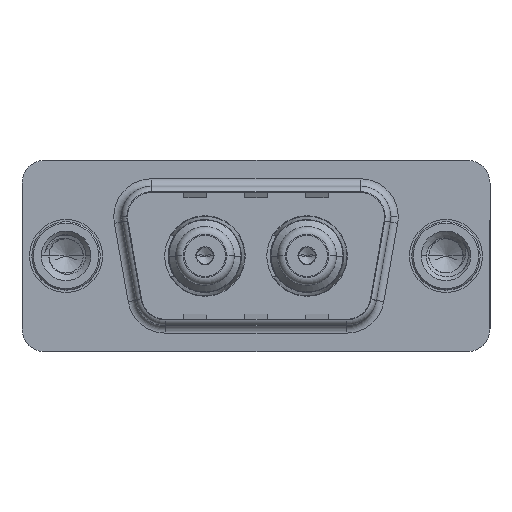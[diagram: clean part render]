
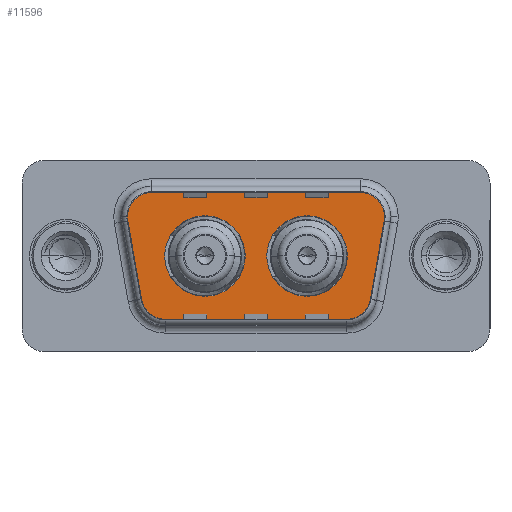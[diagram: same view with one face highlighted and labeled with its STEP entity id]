
A CAD part, top view. The second image highlights one B-rep face of the part: STEP entity #11596.
In plain terms, the highlighted planar face has unit normal (0, 0, 1).
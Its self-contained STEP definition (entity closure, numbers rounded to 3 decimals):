
#60 = DIRECTION ( 'NONE',  ( -1., 0., 0. ) ) ;
#128 = DIRECTION ( 'NONE',  ( 0., 0., 1. ) ) ;
#171 = AXIS2_PLACEMENT_3D ( 'NONE', #3546, #12994, #4929 ) ;
#443 = CARTESIAN_POINT ( 'NONE',  ( 6.459, -4.9, 0. ) ) ;
#576 = CARTESIAN_POINT ( 'NONE',  ( 5.436, 4.9, 0. ) ) ;
#838 = ORIENTED_EDGE ( 'NONE', *, *, #3028, .T. ) ;
#937 = DIRECTION ( 'NONE',  ( 0., 0., 1. ) ) ;
#1273 = DIRECTION ( 'NONE',  ( 0., 0., 1. ) ) ;
#1334 = ORIENTED_EDGE ( 'NONE', *, *, #12226, .F. ) ;
#1441 = VERTEX_POINT ( 'NONE', #5555 ) ;
#1493 = CARTESIAN_POINT ( 'NONE',  ( 20.511, -3.247, 0. ) ) ;
#1774 = ORIENTED_EDGE ( 'NONE', *, *, #13224, .F. ) ;
#1901 = PLANE ( 'NONE',  #8703 ) ;
#2397 = DIRECTION ( 'NONE',  ( 0., 0., 1. ) ) ;
#2769 = CIRCLE ( 'NONE', #3136, 2. ) ;
#2845 = VERTEX_POINT ( 'NONE', #7801 ) ;
#3028 = EDGE_CURVE ( 'NONE', #17390, #1441, #2769, .T. ) ;
#3136 = AXIS2_PLACEMENT_3D ( 'NONE', #5857, #11911, #10556 ) ;
#3280 = CARTESIAN_POINT ( 'NONE',  ( 13.21, 0., 0. ) ) ;
#3546 = CARTESIAN_POINT ( 'NONE',  ( 15.86, 0., 0. ) ) ;
#3594 = EDGE_LOOP ( 'NONE', ( #1774, #10455 ) ) ;
#3660 = ORIENTED_EDGE ( 'NONE', *, *, #9618, .T. ) ;
#4076 = DIRECTION ( 'NONE',  ( 0.174, 0.985, 0. ) ) ;
#4195 = EDGE_CURVE ( 'NONE', #12806, #14596, #5097, .T. ) ;
#4252 = VECTOR ( 'NONE', #12597, 1000. ) ;
#4644 = EDGE_CURVE ( 'NONE', #6173, #17390, #8700, .T. ) ;
#4682 = DIRECTION ( 'NONE',  ( 0., 0., 1. ) ) ;
#4697 = VERTEX_POINT ( 'NONE', #3280 ) ;
#4922 = VERTEX_POINT ( 'NONE', #5548 ) ;
#4929 = DIRECTION ( 'NONE',  ( 1., 0., 0. ) ) ;
#4947 = DIRECTION ( 'NONE',  ( 1., 0., 0. ) ) ;
#5097 = CIRCLE ( 'NONE', #16271, 2. ) ;
#5185 = ORIENTED_EDGE ( 'NONE', *, *, #14272, .T. ) ;
#5450 = EDGE_CURVE ( 'NONE', #14596, #13306, #6565, .T. ) ;
#5460 = CARTESIAN_POINT ( 'NONE',  ( 5.436, 4.9, 0. ) ) ;
#5471 = DIRECTION ( 'NONE',  ( 0.174, -0.985, 0. ) ) ;
#5548 = CARTESIAN_POINT ( 'NONE',  ( 6.459, -4.9, 0. ) ) ;
#5555 = CARTESIAN_POINT ( 'NONE',  ( 19.564, 4.9, 0. ) ) ;
#5847 = AXIS2_PLACEMENT_3D ( 'NONE', #14901, #6826, #16243 ) ;
#5849 = CIRCLE ( 'NONE', #14336, 2.65 ) ;
#5857 = CARTESIAN_POINT ( 'NONE',  ( 19.564, 2.9, 0. ) ) ;
#6173 = VERTEX_POINT ( 'NONE', #9937 ) ;
#6263 = CARTESIAN_POINT ( 'NONE',  ( 3.466, 2.553, 0. ) ) ;
#6487 = FACE_BOUND ( 'NONE', #13799, .T. ) ;
#6512 = ORIENTED_EDGE ( 'NONE', *, *, #14860, .F. ) ;
#6548 = LINE ( 'NONE', #576, #9695 ) ;
#6565 = LINE ( 'NONE', #12731, #9291 ) ;
#6826 = DIRECTION ( 'NONE',  ( 0., 0., 1. ) ) ;
#6878 = DIRECTION ( 'NONE',  ( 0., 0., 1. ) ) ;
#6931 = EDGE_CURVE ( 'NONE', #4922, #2845, #15038, .T. ) ;
#7434 = DIRECTION ( 'NONE',  ( -1., 0., 0. ) ) ;
#7801 = CARTESIAN_POINT ( 'NONE',  ( 18.541, -4.9, 0. ) ) ;
#7809 = VERTEX_POINT ( 'NONE', #1493 ) ;
#8114 = CIRCLE ( 'NONE', #5847, 2.65 ) ;
#8216 = VECTOR ( 'NONE', #4076, 1000. ) ;
#8343 = DIRECTION ( 'NONE',  ( 0., 0., 1. ) ) ;
#8403 = CARTESIAN_POINT ( 'NONE',  ( 15.86, 0., 0. ) ) ;
#8700 = CIRCLE ( 'NONE', #11063, 2. ) ;
#8703 = AXIS2_PLACEMENT_3D ( 'NONE', #11393, #4682, #14122 ) ;
#9019 = CARTESIAN_POINT ( 'NONE',  ( 5.436, 2.9, 0. ) ) ;
#9164 = CARTESIAN_POINT ( 'NONE',  ( 9.14, 0., 0. ) ) ;
#9187 = CARTESIAN_POINT ( 'NONE',  ( 4.489, -3.247, 0. ) ) ;
#9271 = CARTESIAN_POINT ( 'NONE',  ( 18.51, 0., 0. ) ) ;
#9291 = VECTOR ( 'NONE', #5471, 1000. ) ;
#9311 = EDGE_CURVE ( 'NONE', #1441, #12806, #6548, .T. ) ;
#9360 = CARTESIAN_POINT ( 'NONE',  ( 11.79, 0., 0. ) ) ;
#9487 = CARTESIAN_POINT ( 'NONE',  ( 18.541, -2.9, 0. ) ) ;
#9618 = EDGE_CURVE ( 'NONE', #2845, #7809, #17087, .T. ) ;
#9695 = VECTOR ( 'NONE', #7434, 1000. ) ;
#9727 = DIRECTION ( 'NONE',  ( 1., 0., 0. ) ) ;
#9844 = CARTESIAN_POINT ( 'NONE',  ( 21.564, 2.9, 0. ) ) ;
#9905 = ORIENTED_EDGE ( 'NONE', *, *, #6931, .T. ) ;
#9937 = CARTESIAN_POINT ( 'NONE',  ( 21.534, 2.553, 0. ) ) ;
#10294 = EDGE_CURVE ( 'NONE', #7809, #6173, #14941, .T. ) ;
#10455 = ORIENTED_EDGE ( 'NONE', *, *, #15374, .F. ) ;
#10480 = DIRECTION ( 'NONE',  ( 1., 0., 0. ) ) ;
#10542 = CIRCLE ( 'NONE', #14545, 2.65 ) ;
#10556 = DIRECTION ( 'NONE',  ( -1., 0., 0. ) ) ;
#10571 = CARTESIAN_POINT ( 'NONE',  ( 19.564, 2.9, 0. ) ) ;
#10816 = DIRECTION ( 'NONE',  ( 1., 0., 0. ) ) ;
#11060 = ORIENTED_EDGE ( 'NONE', *, *, #4195, .T. ) ;
#11063 = AXIS2_PLACEMENT_3D ( 'NONE', #10571, #6878, #16363 ) ;
#11270 = VERTEX_POINT ( 'NONE', #9360 ) ;
#11326 = CARTESIAN_POINT ( 'NONE',  ( 6.49, 0., 0. ) ) ;
#11393 = CARTESIAN_POINT ( 'NONE',  ( 18.541, -2.9, 0. ) ) ;
#11415 = ORIENTED_EDGE ( 'NONE', *, *, #4644, .T. ) ;
#11596 = ADVANCED_FACE ( 'NONE', ( #16792, #6487, #13192 ), #1901, .T. ) ;
#11909 = CIRCLE ( 'NONE', #171, 2.65 ) ;
#11911 = DIRECTION ( 'NONE',  ( 0., 0., 1. ) ) ;
#12162 = CARTESIAN_POINT ( 'NONE',  ( 21.534, 2.553, 0. ) ) ;
#12226 = EDGE_CURVE ( 'NONE', #15119, #11270, #5849, .T. ) ;
#12597 = DIRECTION ( 'NONE',  ( 1., 0., 0. ) ) ;
#12731 = CARTESIAN_POINT ( 'NONE',  ( 3.466, 2.553, 0. ) ) ;
#12806 = VERTEX_POINT ( 'NONE', #5460 ) ;
#12994 = DIRECTION ( 'NONE',  ( 0., 0., 1. ) ) ;
#13192 = FACE_OUTER_BOUND ( 'NONE', #16115, .T. ) ;
#13224 = EDGE_CURVE ( 'NONE', #14132, #4697, #11909, .T. ) ;
#13306 = VERTEX_POINT ( 'NONE', #9187 ) ;
#13429 = ORIENTED_EDGE ( 'NONE', *, *, #5450, .T. ) ;
#13799 = EDGE_LOOP ( 'NONE', ( #6512, #1334 ) ) ;
#14122 = DIRECTION ( 'NONE',  ( 1., 0., 0. ) ) ;
#14132 = VERTEX_POINT ( 'NONE', #9271 ) ;
#14272 = EDGE_CURVE ( 'NONE', #13306, #4922, #14439, .T. ) ;
#14336 = AXIS2_PLACEMENT_3D ( 'NONE', #9164, #937, #10480 ) ;
#14439 = CIRCLE ( 'NONE', #15875, 2. ) ;
#14545 = AXIS2_PLACEMENT_3D ( 'NONE', #8403, #128, #9727 ) ;
#14596 = VERTEX_POINT ( 'NONE', #6263 ) ;
#14648 = AXIS2_PLACEMENT_3D ( 'NONE', #9487, #1273, #10816 ) ;
#14860 = EDGE_CURVE ( 'NONE', #11270, #15119, #8114, .T. ) ;
#14901 = CARTESIAN_POINT ( 'NONE',  ( 9.14, 0., 0. ) ) ;
#14941 = LINE ( 'NONE', #12162, #8216 ) ;
#15038 = LINE ( 'NONE', #443, #4252 ) ;
#15119 = VERTEX_POINT ( 'NONE', #11326 ) ;
#15221 = ORIENTED_EDGE ( 'NONE', *, *, #10294, .T. ) ;
#15308 = ORIENTED_EDGE ( 'NONE', *, *, #9311, .T. ) ;
#15374 = EDGE_CURVE ( 'NONE', #4697, #14132, #10542, .T. ) ;
#15875 = AXIS2_PLACEMENT_3D ( 'NONE', #16388, #8343, #60 ) ;
#16115 = EDGE_LOOP ( 'NONE', ( #3660, #15221, #11415, #838, #15308, #11060, #13429, #5185, #9905 ) ) ;
#16243 = DIRECTION ( 'NONE',  ( 1., 0., 0. ) ) ;
#16271 = AXIS2_PLACEMENT_3D ( 'NONE', #9019, #2397, #4947 ) ;
#16363 = DIRECTION ( 'NONE',  ( -1., 0., 0. ) ) ;
#16388 = CARTESIAN_POINT ( 'NONE',  ( 6.459, -2.9, 0. ) ) ;
#16792 = FACE_BOUND ( 'NONE', #3594, .T. ) ;
#17087 = CIRCLE ( 'NONE', #14648, 2. ) ;
#17390 = VERTEX_POINT ( 'NONE', #9844 ) ;
